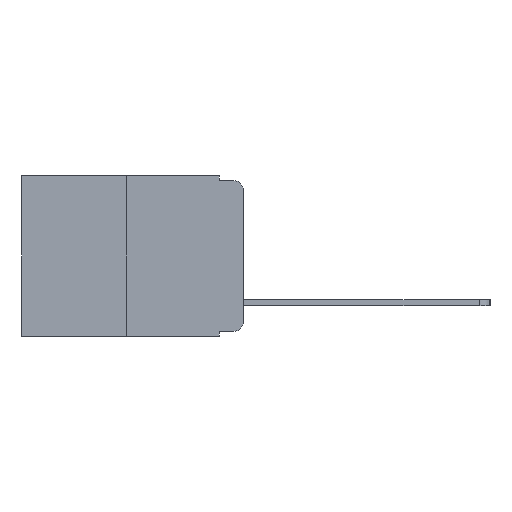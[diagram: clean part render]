
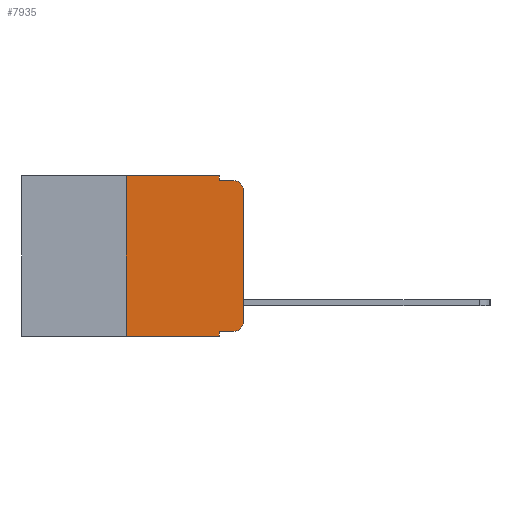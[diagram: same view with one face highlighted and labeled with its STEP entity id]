
A CAD part, left-side view. The second image highlights one B-rep face of the part: STEP entity #7935.
In plain terms, the highlighted planar face has unit normal (-1, 0, 0).
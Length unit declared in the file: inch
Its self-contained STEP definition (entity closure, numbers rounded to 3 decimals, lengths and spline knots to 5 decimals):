
#2 = ORIENTED_EDGE ( 'NONE', *, *, #8499, .F. ) ;
#73 = CARTESIAN_POINT ( 'NONE',  ( 0., 0.25, 0. ) ) ;
#394 = VECTOR ( 'NONE', #8989, 39.37008 ) ;
#508 = AXIS2_PLACEMENT_3D ( 'NONE', #6909, #943, #7837 ) ;
#892 = EDGE_LOOP ( 'NONE', ( #4348, #9792, #7760, #2, #8897, #2801, #1332, #12038, #3236, #10802 ) ) ;
#937 = AXIS2_PLACEMENT_3D ( 'NONE', #8678, #2947, #9608 ) ;
#943 = DIRECTION ( 'NONE',  ( -1., 0., 0. ) ) ;
#1147 = DIRECTION ( 'NONE',  ( 0., -1., 0. ) ) ;
#1295 = VECTOR ( 'NONE', #11450, 39.37008 ) ;
#1304 = LINE ( 'NONE', #7239, #10935 ) ;
#1332 = ORIENTED_EDGE ( 'NONE', *, *, #3975, .T. ) ;
#1994 = DIRECTION ( 'NONE',  ( 0., -1., 0. ) ) ;
#2416 = VECTOR ( 'NONE', #5226, 39.37008 ) ;
#2801 = ORIENTED_EDGE ( 'NONE', *, *, #4464, .F. ) ;
#2903 = CARTESIAN_POINT ( 'NONE',  ( 0., 0.051, -0.01 ) ) ;
#2947 = DIRECTION ( 'NONE',  ( -1., 0., 0. ) ) ;
#3082 = VERTEX_POINT ( 'NONE', #4257 ) ;
#3236 = ORIENTED_EDGE ( 'NONE', *, *, #10754, .T. ) ;
#3264 = LINE ( 'NONE', #8921, #394 ) ;
#3610 = VERTEX_POINT ( 'NONE', #6744 ) ;
#3911 = CARTESIAN_POINT ( 'NONE',  ( 0., 0., -0.313 ) ) ;
#3953 = CARTESIAN_POINT ( 'NONE',  ( 0., 0.051, 0. ) ) ;
#3975 = EDGE_CURVE ( 'NONE', #5802, #6438, #12330, .T. ) ;
#3989 = PLANE ( 'NONE',  #6873 ) ;
#4257 = CARTESIAN_POINT ( 'NONE',  ( 0., 0.02, -0.01 ) ) ;
#4348 = ORIENTED_EDGE ( 'NONE', *, *, #10131, .T. ) ;
#4444 = VERTEX_POINT ( 'NONE', #9762 ) ;
#4464 = EDGE_CURVE ( 'NONE', #5802, #6537, #3264, .T. ) ;
#4653 = CARTESIAN_POINT ( 'NONE',  ( 0., 0.051, 0. ) ) ;
#4837 = VECTOR ( 'NONE', #1994, 39.37008 ) ;
#4887 = CARTESIAN_POINT ( 'NONE',  ( 0., 0.473, -0.343 ) ) ;
#4952 = CARTESIAN_POINT ( 'NONE',  ( 0., 0.473, 0. ) ) ;
#5071 = LINE ( 'NONE', #6171, #2416 ) ;
#5095 = CIRCLE ( 'NONE', #937, 0.02 ) ;
#5226 = DIRECTION ( 'NONE',  ( 0., -1., 0. ) ) ;
#5373 = LINE ( 'NONE', #4653, #11374 ) ;
#5479 = CARTESIAN_POINT ( 'NONE',  ( 0., 0.051, -0.01 ) ) ;
#5731 = EDGE_CURVE ( 'NONE', #11225, #3082, #10535, .T. ) ;
#5802 = VERTEX_POINT ( 'NONE', #8812 ) ;
#5807 = LINE ( 'NONE', #12688, #10790 ) ;
#5923 = DIRECTION ( 'NONE',  ( 1., 0., 0. ) ) ;
#5944 = FACE_OUTER_BOUND ( 'NONE', #892, .T. ) ;
#6171 = CARTESIAN_POINT ( 'NONE',  ( 0., 0.051, -0.333 ) ) ;
#6245 = VERTEX_POINT ( 'NONE', #3953 ) ;
#6246 = LINE ( 'NONE', #12282, #11498 ) ;
#6438 = VERTEX_POINT ( 'NONE', #8877 ) ;
#6537 = VERTEX_POINT ( 'NONE', #73 ) ;
#6662 = DIRECTION ( 'NONE',  ( 0., 0., -1. ) ) ;
#6744 = CARTESIAN_POINT ( 'NONE',  ( 0., 0.02, -0.333 ) ) ;
#6873 = AXIS2_PLACEMENT_3D ( 'NONE', #4952, #5923, #12500 ) ;
#6909 = CARTESIAN_POINT ( 'NONE',  ( 0., 0.02, -0.03 ) ) ;
#7016 = EDGE_CURVE ( 'NONE', #3610, #12713, #5095, .T. ) ;
#7239 = CARTESIAN_POINT ( 'NONE',  ( 0., 0., 0. ) ) ;
#7556 = VERTEX_POINT ( 'NONE', #5479 ) ;
#7636 = EDGE_CURVE ( 'NONE', #4444, #6438, #5373, .T. ) ;
#7753 = CARTESIAN_POINT ( 'NONE',  ( 0., 0., -0.03 ) ) ;
#7760 = ORIENTED_EDGE ( 'NONE', *, *, #7864, .F. ) ;
#7837 = DIRECTION ( 'NONE',  ( 0., 0., -1. ) ) ;
#7864 = EDGE_CURVE ( 'NONE', #7556, #3082, #9026, .T. ) ;
#7935 = ADVANCED_FACE ( 'NONE', ( #5944 ), #3989, .F. ) ;
#8499 = EDGE_CURVE ( 'NONE', #6245, #7556, #6246, .T. ) ;
#8678 = CARTESIAN_POINT ( 'NONE',  ( 0., 0.02, -0.313 ) ) ;
#8812 = CARTESIAN_POINT ( 'NONE',  ( 0., 0.25, -0.343 ) ) ;
#8877 = CARTESIAN_POINT ( 'NONE',  ( 0., 0.051, -0.343 ) ) ;
#8897 = ORIENTED_EDGE ( 'NONE', *, *, #9366, .F. ) ;
#8921 = CARTESIAN_POINT ( 'NONE',  ( 0., 0.25, 0. ) ) ;
#8989 = DIRECTION ( 'NONE',  ( 0., 0., 1. ) ) ;
#9026 = LINE ( 'NONE', #2903, #1295 ) ;
#9366 = EDGE_CURVE ( 'NONE', #6537, #6245, #5807, .T. ) ;
#9608 = DIRECTION ( 'NONE',  ( 0., 0., -1. ) ) ;
#9762 = CARTESIAN_POINT ( 'NONE',  ( 0., 0.051, -0.333 ) ) ;
#9792 = ORIENTED_EDGE ( 'NONE', *, *, #5731, .T. ) ;
#10131 = EDGE_CURVE ( 'NONE', #12713, #11225, #1304, .T. ) ;
#10535 = CIRCLE ( 'NONE', #508, 0.02 ) ;
#10754 = EDGE_CURVE ( 'NONE', #4444, #3610, #5071, .T. ) ;
#10790 = VECTOR ( 'NONE', #1147, 39.37008 ) ;
#10802 = ORIENTED_EDGE ( 'NONE', *, *, #7016, .T. ) ;
#10935 = VECTOR ( 'NONE', #11889, 39.37008 ) ;
#11199 = DIRECTION ( 'NONE',  ( 0., 0., -1. ) ) ;
#11225 = VERTEX_POINT ( 'NONE', #7753 ) ;
#11374 = VECTOR ( 'NONE', #11199, 39.37008 ) ;
#11450 = DIRECTION ( 'NONE',  ( 0., -1., 0. ) ) ;
#11498 = VECTOR ( 'NONE', #6662, 39.37008 ) ;
#11889 = DIRECTION ( 'NONE',  ( 0., 0., 1. ) ) ;
#12038 = ORIENTED_EDGE ( 'NONE', *, *, #7636, .F. ) ;
#12282 = CARTESIAN_POINT ( 'NONE',  ( 0., 0.051, 0. ) ) ;
#12330 = LINE ( 'NONE', #4887, #4837 ) ;
#12500 = DIRECTION ( 'NONE',  ( 0., 0., -1. ) ) ;
#12688 = CARTESIAN_POINT ( 'NONE',  ( 0., 0.473, 0. ) ) ;
#12713 = VERTEX_POINT ( 'NONE', #3911 ) ;
